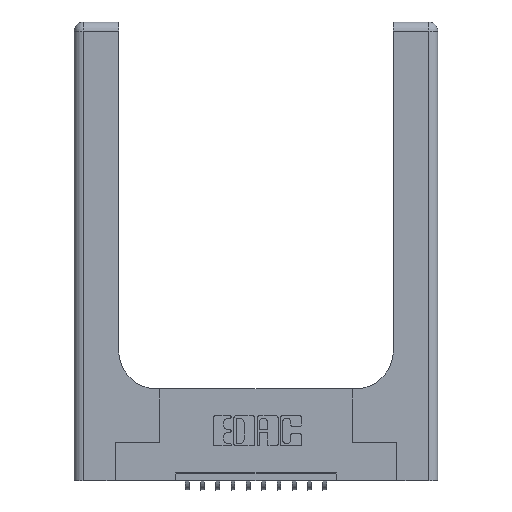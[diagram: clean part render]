
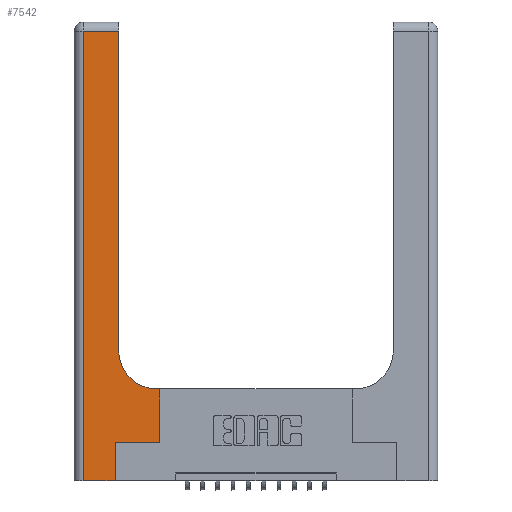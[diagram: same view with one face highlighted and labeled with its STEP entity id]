
A CAD part, top view. The second image highlights one B-rep face of the part: STEP entity #7542.
In plain terms, the highlighted planar face has unit normal (0, 0, 1).
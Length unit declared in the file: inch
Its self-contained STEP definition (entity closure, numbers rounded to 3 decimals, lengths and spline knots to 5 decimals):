
#540 = CARTESIAN_POINT ( 'NONE',  ( 0.5415, 0.85, 0.37 ) ) ;
#644 = DIRECTION ( 'NONE',  ( 1., 0., 0. ) ) ;
#730 = CARTESIAN_POINT ( 'NONE',  ( 0., 3., 0.37 ) ) ;
#945 = LINE ( 'NONE', #10460, #7582 ) ;
#1239 = CIRCLE ( 'NONE', #3918, 0.25 ) ;
#1392 = CARTESIAN_POINT ( 'NONE',  ( 0.269, 0.25, 0.37 ) ) ;
#1786 = CARTESIAN_POINT ( 'NONE',  ( 0.06, 0., 0.37 ) ) ;
#2162 = EDGE_CURVE ( 'NONE', #12119, #16435, #5120, .T. ) ;
#2186 = VERTEX_POINT ( 'NONE', #11722 ) ;
#2314 = ORIENTED_EDGE ( 'NONE', *, *, #2162, .T. ) ;
#3103 = VECTOR ( 'NONE', #644, 39.37008 ) ;
#3589 = LINE ( 'NONE', #8498, #5221 ) ;
#3612 = VERTEX_POINT ( 'NONE', #1392 ) ;
#3682 = ORIENTED_EDGE ( 'NONE', *, *, #14575, .T. ) ;
#3763 = ORIENTED_EDGE ( 'NONE', *, *, #5911, .T. ) ;
#3918 = AXIS2_PLACEMENT_3D ( 'NONE', #540, #5696, #11016 ) ;
#4470 = VERTEX_POINT ( 'NONE', #10391 ) ;
#4577 = VERTEX_POINT ( 'NONE', #16735 ) ;
#4858 = VECTOR ( 'NONE', #12588, 39.37008 ) ;
#5120 = LINE ( 'NONE', #6348, #14425 ) ;
#5221 = VECTOR ( 'NONE', #8371, 39.37008 ) ;
#5458 = VECTOR ( 'NONE', #16748, 39.37008 ) ;
#5696 = DIRECTION ( 'NONE',  ( 0., 0., -1. ) ) ;
#5816 = EDGE_CURVE ( 'NONE', #2186, #4577, #1239, .T. ) ;
#5911 = EDGE_CURVE ( 'NONE', #6585, #16107, #14481, .T. ) ;
#6348 = CARTESIAN_POINT ( 'NONE',  ( 0., 2.94, 0.37 ) ) ;
#6351 = FACE_OUTER_BOUND ( 'NONE', #15366, .T. ) ;
#6463 = DIRECTION ( 'NONE',  ( -1., 0., 0. ) ) ;
#6467 = CARTESIAN_POINT ( 'NONE',  ( 0.2915, 3., 0.37 ) ) ;
#6496 = LINE ( 'NONE', #8798, #5458 ) ;
#6547 = CARTESIAN_POINT ( 'NONE',  ( 0.269, 0., 0.37 ) ) ;
#6585 = VERTEX_POINT ( 'NONE', #1786 ) ;
#7405 = DIRECTION ( 'NONE',  ( 0., 0., -1. ) ) ;
#7542 = ADVANCED_FACE ( 'NONE', ( #6351 ), #15262, .F. ) ;
#7548 = LINE ( 'NONE', #13854, #4858 ) ;
#7582 = VECTOR ( 'NONE', #8353, 39.37008 ) ;
#7834 = ORIENTED_EDGE ( 'NONE', *, *, #14188, .T. ) ;
#8306 = CARTESIAN_POINT ( 'NONE',  ( 0.06, 2.94, 0.37 ) ) ;
#8353 = DIRECTION ( 'NONE',  ( 1., 0., 0. ) ) ;
#8371 = DIRECTION ( 'NONE',  ( -1., 0., 0. ) ) ;
#8459 = AXIS2_PLACEMENT_3D ( 'NONE', #730, #7405, #16618 ) ;
#8498 = CARTESIAN_POINT ( 'NONE',  ( 0.2915, 0.6, 0.37 ) ) ;
#8798 = CARTESIAN_POINT ( 'NONE',  ( 0.06, 3., 0.37 ) ) ;
#8822 = CARTESIAN_POINT ( 'NONE',  ( 0.5585, 0.6, 0.37 ) ) ;
#8972 = VECTOR ( 'NONE', #11805, 39.37008 ) ;
#9173 = VERTEX_POINT ( 'NONE', #8822 ) ;
#9833 = LINE ( 'NONE', #6467, #17040 ) ;
#9986 = LINE ( 'NONE', #6547, #8972 ) ;
#10077 = ORIENTED_EDGE ( 'NONE', *, *, #16091, .T. ) ;
#10080 = ORIENTED_EDGE ( 'NONE', *, *, #13603, .T. ) ;
#10391 = CARTESIAN_POINT ( 'NONE',  ( 0.5585, 0.25, 0.37 ) ) ;
#10460 = CARTESIAN_POINT ( 'NONE',  ( 0.269, 0.25, 0.37 ) ) ;
#11016 = DIRECTION ( 'NONE',  ( 1., 0., 0. ) ) ;
#11395 = CARTESIAN_POINT ( 'NONE',  ( 0.269, 0., 0.37 ) ) ;
#11722 = CARTESIAN_POINT ( 'NONE',  ( 0.5415, 0.6, 0.37 ) ) ;
#11805 = DIRECTION ( 'NONE',  ( 0., 1., 0. ) ) ;
#12045 = EDGE_CURVE ( 'NONE', #9173, #2186, #3589, .T. ) ;
#12119 = VERTEX_POINT ( 'NONE', #12420 ) ;
#12420 = CARTESIAN_POINT ( 'NONE',  ( 0.2915, 2.94, 0.37 ) ) ;
#12588 = DIRECTION ( 'NONE',  ( 0., 1., 0. ) ) ;
#13051 = ORIENTED_EDGE ( 'NONE', *, *, #5816, .T. ) ;
#13603 = EDGE_CURVE ( 'NONE', #3612, #4470, #945, .T. ) ;
#13854 = CARTESIAN_POINT ( 'NONE',  ( 0.5585, 0.25, 0.37 ) ) ;
#14188 = EDGE_CURVE ( 'NONE', #4577, #12119, #9833, .T. ) ;
#14425 = VECTOR ( 'NONE', #6463, 39.37008 ) ;
#14481 = LINE ( 'NONE', #15291, #3103 ) ;
#14575 = EDGE_CURVE ( 'NONE', #4470, #9173, #7548, .T. ) ;
#15262 = PLANE ( 'NONE',  #8459 ) ;
#15291 = CARTESIAN_POINT ( 'NONE',  ( 0., 0., 0.37 ) ) ;
#15366 = EDGE_LOOP ( 'NONE', ( #7834, #2314, #10077, #3763, #16156, #10080, #3682, #16398, #13051 ) ) ;
#15631 = DIRECTION ( 'NONE',  ( 0., 1., 0. ) ) ;
#16091 = EDGE_CURVE ( 'NONE', #16435, #6585, #6496, .T. ) ;
#16107 = VERTEX_POINT ( 'NONE', #11395 ) ;
#16156 = ORIENTED_EDGE ( 'NONE', *, *, #16206, .T. ) ;
#16206 = EDGE_CURVE ( 'NONE', #16107, #3612, #9986, .T. ) ;
#16398 = ORIENTED_EDGE ( 'NONE', *, *, #12045, .T. ) ;
#16435 = VERTEX_POINT ( 'NONE', #8306 ) ;
#16618 = DIRECTION ( 'NONE',  ( -1., 0., 0. ) ) ;
#16735 = CARTESIAN_POINT ( 'NONE',  ( 0.2915, 0.85, 0.37 ) ) ;
#16748 = DIRECTION ( 'NONE',  ( 0., -1., 0. ) ) ;
#17040 = VECTOR ( 'NONE', #15631, 39.37008 ) ;
